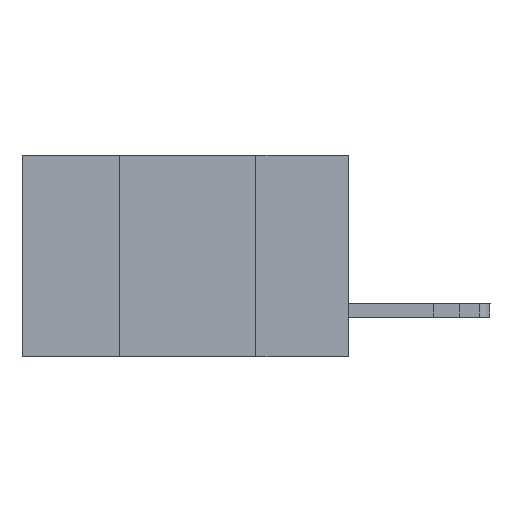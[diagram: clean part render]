
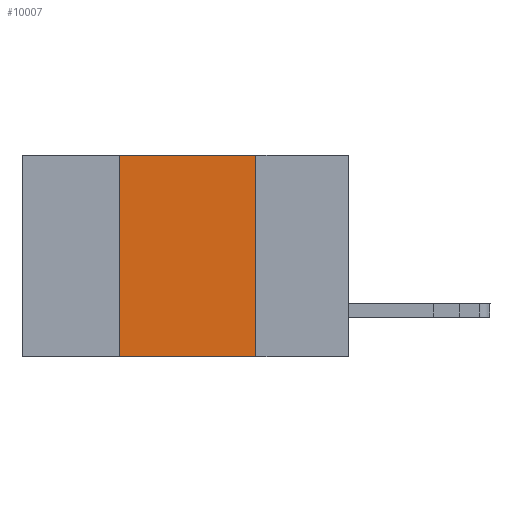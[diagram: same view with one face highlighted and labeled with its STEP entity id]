
A CAD part, left-side view. The second image highlights one B-rep face of the part: STEP entity #10007.
In plain terms, the highlighted planar face has unit normal (-1, 0, 0).
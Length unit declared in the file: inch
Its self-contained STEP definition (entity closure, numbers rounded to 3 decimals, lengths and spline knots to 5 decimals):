
#1198 = CARTESIAN_POINT ( 'NONE',  ( 0., 0.17, -0.37 ) ) ;
#1679 = VECTOR ( 'NONE', #3481, 39.37008 ) ;
#2117 = ORIENTED_EDGE ( 'NONE', *, *, #2254, .F. ) ;
#2254 = EDGE_CURVE ( 'NONE', #11554, #8509, #10192, .T. ) ;
#2465 = DIRECTION ( 'NONE',  ( 0., -1., 0. ) ) ;
#2834 = CARTESIAN_POINT ( 'NONE',  ( 0., 0.6, 0. ) ) ;
#2888 = VECTOR ( 'NONE', #3913, 39.37008 ) ;
#3024 = CARTESIAN_POINT ( 'NONE',  ( 0., 0.42, -0.37 ) ) ;
#3425 = CARTESIAN_POINT ( 'NONE',  ( 0., 0.17, -0.37 ) ) ;
#3481 = DIRECTION ( 'NONE',  ( 0., 0., -1. ) ) ;
#3566 = DIRECTION ( 'NONE',  ( 0., -1., 0. ) ) ;
#3913 = DIRECTION ( 'NONE',  ( 0., 0., 1. ) ) ;
#4250 = EDGE_CURVE ( 'NONE', #8654, #8509, #5580, .T. ) ;
#4996 = PLANE ( 'NONE',  #12178 ) ;
#5546 = CARTESIAN_POINT ( 'NONE',  ( 0., 0.42, -0.37 ) ) ;
#5580 = LINE ( 'NONE', #10456, #5957 ) ;
#5957 = VECTOR ( 'NONE', #3566, 39.37008 ) ;
#6047 = ORIENTED_EDGE ( 'NONE', *, *, #10053, .F. ) ;
#6312 = LINE ( 'NONE', #11179, #8818 ) ;
#6467 = ORIENTED_EDGE ( 'NONE', *, *, #4250, .T. ) ;
#6881 = FACE_OUTER_BOUND ( 'NONE', #10404, .T. ) ;
#7070 = VERTEX_POINT ( 'NONE', #10752 ) ;
#7255 = EDGE_CURVE ( 'NONE', #7070, #11554, #6312, .T. ) ;
#8509 = VERTEX_POINT ( 'NONE', #1198 ) ;
#8654 = VERTEX_POINT ( 'NONE', #5546 ) ;
#8818 = VECTOR ( 'NONE', #2465, 39.37008 ) ;
#9537 = DIRECTION ( 'NONE',  ( 1., 0., 0. ) ) ;
#10007 = ADVANCED_FACE ( 'NONE', ( #6881 ), #4996, .F. ) ;
#10053 = EDGE_CURVE ( 'NONE', #8654, #7070, #10547, .T. ) ;
#10082 = ORIENTED_EDGE ( 'NONE', *, *, #7255, .F. ) ;
#10192 = LINE ( 'NONE', #3425, #1679 ) ;
#10404 = EDGE_LOOP ( 'NONE', ( #2117, #10082, #6047, #6467 ) ) ;
#10456 = CARTESIAN_POINT ( 'NONE',  ( 0., 0.6, -0.37 ) ) ;
#10547 = LINE ( 'NONE', #3024, #2888 ) ;
#10752 = CARTESIAN_POINT ( 'NONE',  ( 0., 0.42, 0. ) ) ;
#11179 = CARTESIAN_POINT ( 'NONE',  ( 0., 0.6, 0. ) ) ;
#11554 = VERTEX_POINT ( 'NONE', #11851 ) ;
#11686 = DIRECTION ( 'NONE',  ( 0., 0., -1. ) ) ;
#11851 = CARTESIAN_POINT ( 'NONE',  ( 0., 0.17, 0. ) ) ;
#12178 = AXIS2_PLACEMENT_3D ( 'NONE', #2834, #9537, #11686 ) ;
